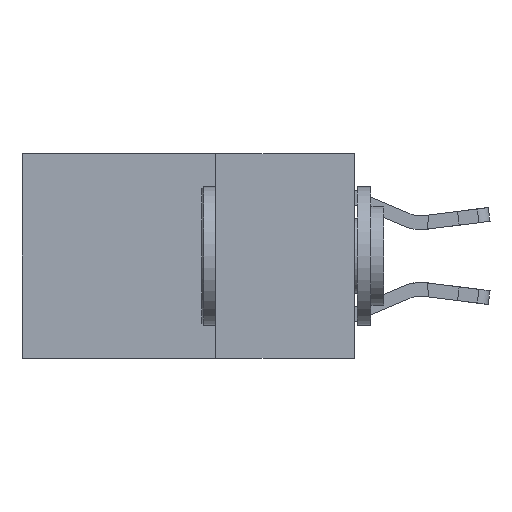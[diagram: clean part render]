
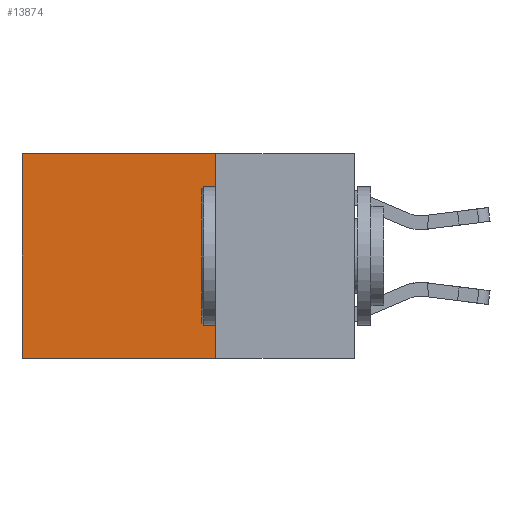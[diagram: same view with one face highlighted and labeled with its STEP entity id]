
A CAD part, left-side view. The second image highlights one B-rep face of the part: STEP entity #13874.
In plain terms, the highlighted planar face has unit normal (-1, 0, 0).
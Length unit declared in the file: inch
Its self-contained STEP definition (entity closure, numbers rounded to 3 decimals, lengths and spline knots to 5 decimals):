
#1193 = EDGE_LOOP ( 'NONE', ( #4078, #7159, #5094, #1635 ) ) ;
#1635 = ORIENTED_EDGE ( 'NONE', *, *, #7978, .T. ) ;
#2143 = DIRECTION ( 'NONE',  ( 0., 0., -1. ) ) ;
#2398 = CARTESIAN_POINT ( 'NONE',  ( 0.2625, 0.6, 0. ) ) ;
#2413 = DIRECTION ( 'NONE',  ( 1., 0., 0. ) ) ;
#3103 = CARTESIAN_POINT ( 'NONE',  ( 0.2625, 0.6, 0. ) ) ;
#4078 = ORIENTED_EDGE ( 'NONE', *, *, #10229, .T. ) ;
#4306 = DIRECTION ( 'NONE',  ( 0., 1., 0. ) ) ;
#4415 = CARTESIAN_POINT ( 'NONE',  ( 0.2625, 0.25, -0.37 ) ) ;
#4433 = DIRECTION ( 'NONE',  ( 0., 0., -1. ) ) ;
#5094 = ORIENTED_EDGE ( 'NONE', *, *, #7044, .F. ) ;
#5310 = CARTESIAN_POINT ( 'NONE',  ( 0.2625, 0.25, -0.37 ) ) ;
#5469 = VERTEX_POINT ( 'NONE', #2398 ) ;
#5648 = VECTOR ( 'NONE', #4433, 39.37008 ) ;
#7044 = EDGE_CURVE ( 'NONE', #16012, #7352, #8499, .T. ) ;
#7077 = CARTESIAN_POINT ( 'NONE',  ( 0.2625, 0.25, 0. ) ) ;
#7159 = ORIENTED_EDGE ( 'NONE', *, *, #10029, .F. ) ;
#7352 = VERTEX_POINT ( 'NONE', #5310 ) ;
#7978 = EDGE_CURVE ( 'NONE', #16012, #5469, #11010, .T. ) ;
#8499 = LINE ( 'NONE', #7077, #5648 ) ;
#8956 = CARTESIAN_POINT ( 'NONE',  ( 0.2625, 0.25, 0. ) ) ;
#9042 = VERTEX_POINT ( 'NONE', #15818 ) ;
#9074 = CARTESIAN_POINT ( 'NONE',  ( 0.2625, 0.25, 0. ) ) ;
#9216 = VECTOR ( 'NONE', #12712, 39.37008 ) ;
#9781 = VECTOR ( 'NONE', #4306, 39.37008 ) ;
#10029 = EDGE_CURVE ( 'NONE', #7352, #9042, #16285, .T. ) ;
#10229 = EDGE_CURVE ( 'NONE', #5469, #9042, #11379, .T. ) ;
#11010 = LINE ( 'NONE', #8956, #9781 ) ;
#11037 = DIRECTION ( 'NONE',  ( 0., 1., 0. ) ) ;
#11379 = LINE ( 'NONE', #3103, #9216 ) ;
#11524 = AXIS2_PLACEMENT_3D ( 'NONE', #15650, #2413, #2143 ) ;
#11555 = PLANE ( 'NONE',  #11524 ) ;
#12712 = DIRECTION ( 'NONE',  ( 0., 0., -1. ) ) ;
#13874 = ADVANCED_FACE ( 'NONE', ( #14571 ), #11555, .F. ) ;
#14571 = FACE_OUTER_BOUND ( 'NONE', #1193, .T. ) ;
#15650 = CARTESIAN_POINT ( 'NONE',  ( 0.2625, 0.25, 0. ) ) ;
#15818 = CARTESIAN_POINT ( 'NONE',  ( 0.2625, 0.6, -0.37 ) ) ;
#16012 = VERTEX_POINT ( 'NONE', #9074 ) ;
#16285 = LINE ( 'NONE', #4415, #17412 ) ;
#17412 = VECTOR ( 'NONE', #11037, 39.37008 ) ;
